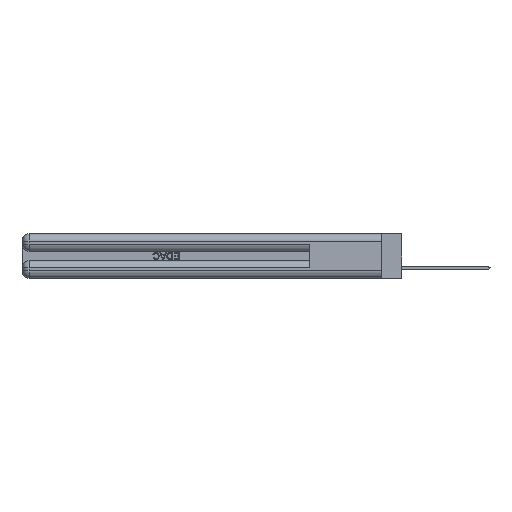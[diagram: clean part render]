
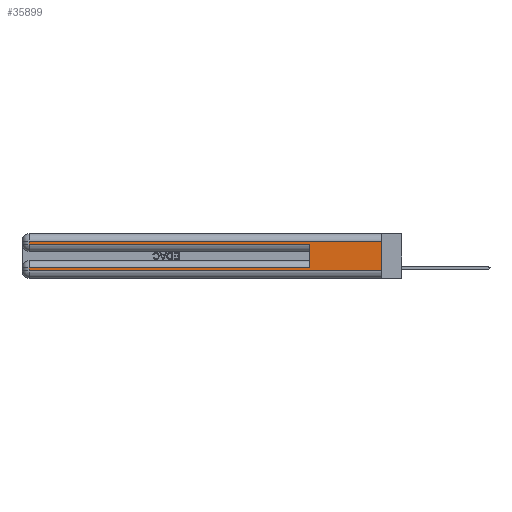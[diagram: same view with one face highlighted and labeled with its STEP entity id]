
A CAD part, left-side view. The second image highlights one B-rep face of the part: STEP entity #35899.
In plain terms, the highlighted planar face has unit normal (-1, 0, 0).
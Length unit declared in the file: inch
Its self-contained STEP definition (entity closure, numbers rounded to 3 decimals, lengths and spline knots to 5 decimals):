
#973 = EDGE_CURVE ( 'NONE', #20612, #2213, #20601, .T. ) ;
#2097 = ORIENTED_EDGE ( 'NONE', *, *, #22844, .T. ) ;
#2213 = VERTEX_POINT ( 'NONE', #9539 ) ;
#3078 = CARTESIAN_POINT ( 'NONE',  ( 0., 0.6, 0.285 ) ) ;
#3128 = DIRECTION ( 'NONE',  ( 0., 1., 0. ) ) ;
#4346 = ORIENTED_EDGE ( 'NONE', *, *, #6874, .T. ) ;
#4653 = ORIENTED_EDGE ( 'NONE', *, *, #14646, .T. ) ;
#4677 = DIRECTION ( 'NONE',  ( 0., 0., -1. ) ) ;
#4968 = AXIS2_PLACEMENT_3D ( 'NONE', #41780, #44634, #24439 ) ;
#5576 = VERTEX_POINT ( 'NONE', #21623 ) ;
#5608 = LINE ( 'NONE', #22154, #29517 ) ;
#6390 = VERTEX_POINT ( 'NONE', #28994 ) ;
#6874 = EDGE_CURVE ( 'NONE', #6390, #2213, #15144, .T. ) ;
#8051 = VECTOR ( 'NONE', #33390, 39.37008 ) ;
#8951 = CARTESIAN_POINT ( 'NONE',  ( 0., 0.6, 0.145 ) ) ;
#9172 = VECTOR ( 'NONE', #40538, 39.37008 ) ;
#9253 = DIRECTION ( 'NONE',  ( 0., 0., -1. ) ) ;
#9539 = CARTESIAN_POINT ( 'NONE',  ( 0., 0., 0.06 ) ) ;
#11825 = CARTESIAN_POINT ( 'NONE',  ( 0., 2.94, 0.37 ) ) ;
#12664 = EDGE_CURVE ( 'NONE', #20612, #14022, #36190, .T. ) ;
#12859 = LINE ( 'NONE', #11825, #23737 ) ;
#12977 = CARTESIAN_POINT ( 'NONE',  ( 0., 0., 0.31 ) ) ;
#13374 = VECTOR ( 'NONE', #22067, 39.37008 ) ;
#13629 = PLANE ( 'NONE',  #4968 ) ;
#14022 = VERTEX_POINT ( 'NONE', #27648 ) ;
#14646 = EDGE_CURVE ( 'NONE', #17563, #6390, #5608, .T. ) ;
#15144 = LINE ( 'NONE', #42811, #9172 ) ;
#17334 = LINE ( 'NONE', #8951, #8051 ) ;
#17563 = VERTEX_POINT ( 'NONE', #39526 ) ;
#17765 = CARTESIAN_POINT ( 'NONE',  ( 0., 0., 0.285 ) ) ;
#18097 = EDGE_CURVE ( 'NONE', #5576, #22923, #32224, .T. ) ;
#18388 = EDGE_LOOP ( 'NONE', ( #40863, #36139, #32761, #39510, #37379, #2097, #4653, #4346 ) ) ;
#18585 = CARTESIAN_POINT ( 'NONE',  ( 0., 0., 0.31 ) ) ;
#20601 = LINE ( 'NONE', #30076, #27118 ) ;
#20612 = VERTEX_POINT ( 'NONE', #12977 ) ;
#20699 = EDGE_CURVE ( 'NONE', #29252, #22923, #17334, .T. ) ;
#21623 = CARTESIAN_POINT ( 'NONE',  ( 0., 2.94, 0.285 ) ) ;
#22067 = DIRECTION ( 'NONE',  ( 0., 1., 0. ) ) ;
#22154 = CARTESIAN_POINT ( 'NONE',  ( 0., 2.94, 0.37 ) ) ;
#22844 = EDGE_CURVE ( 'NONE', #29252, #17563, #34472, .T. ) ;
#22923 = VERTEX_POINT ( 'NONE', #3078 ) ;
#23737 = VECTOR ( 'NONE', #27045, 39.37008 ) ;
#24439 = DIRECTION ( 'NONE',  ( 0., 0., -1. ) ) ;
#24798 = EDGE_CURVE ( 'NONE', #14022, #5576, #12859, .T. ) ;
#27045 = DIRECTION ( 'NONE',  ( 0., 0., -1. ) ) ;
#27118 = VECTOR ( 'NONE', #9253, 39.37008 ) ;
#27648 = CARTESIAN_POINT ( 'NONE',  ( 0., 2.94, 0.31 ) ) ;
#28992 = FACE_OUTER_BOUND ( 'NONE', #18388, .T. ) ;
#28994 = CARTESIAN_POINT ( 'NONE',  ( 0., 2.94, 0.06 ) ) ;
#29252 = VERTEX_POINT ( 'NONE', #31528 ) ;
#29517 = VECTOR ( 'NONE', #4677, 39.37008 ) ;
#30076 = CARTESIAN_POINT ( 'NONE',  ( 0., 0., 0.37 ) ) ;
#31130 = VECTOR ( 'NONE', #38298, 39.37008 ) ;
#31528 = CARTESIAN_POINT ( 'NONE',  ( 0., 0.6, 0.085 ) ) ;
#32224 = LINE ( 'NONE', #17765, #31130 ) ;
#32761 = ORIENTED_EDGE ( 'NONE', *, *, #24798, .T. ) ;
#33390 = DIRECTION ( 'NONE',  ( 0., 0., 1. ) ) ;
#34472 = LINE ( 'NONE', #41566, #44662 ) ;
#35899 = ADVANCED_FACE ( 'NONE', ( #28992 ), #13629, .F. ) ;
#36139 = ORIENTED_EDGE ( 'NONE', *, *, #12664, .T. ) ;
#36190 = LINE ( 'NONE', #18585, #13374 ) ;
#37379 = ORIENTED_EDGE ( 'NONE', *, *, #20699, .F. ) ;
#38298 = DIRECTION ( 'NONE',  ( 0., -1., 0. ) ) ;
#39510 = ORIENTED_EDGE ( 'NONE', *, *, #18097, .T. ) ;
#39526 = CARTESIAN_POINT ( 'NONE',  ( 0., 2.94, 0.085 ) ) ;
#40538 = DIRECTION ( 'NONE',  ( 0., -1., 0. ) ) ;
#40863 = ORIENTED_EDGE ( 'NONE', *, *, #973, .F. ) ;
#41566 = CARTESIAN_POINT ( 'NONE',  ( 0., 0., 0.085 ) ) ;
#41780 = CARTESIAN_POINT ( 'NONE',  ( 0., 0., 0.37 ) ) ;
#42811 = CARTESIAN_POINT ( 'NONE',  ( 0., 0., 0.06 ) ) ;
#44634 = DIRECTION ( 'NONE',  ( 1., 0., 0. ) ) ;
#44662 = VECTOR ( 'NONE', #3128, 39.37008 ) ;
